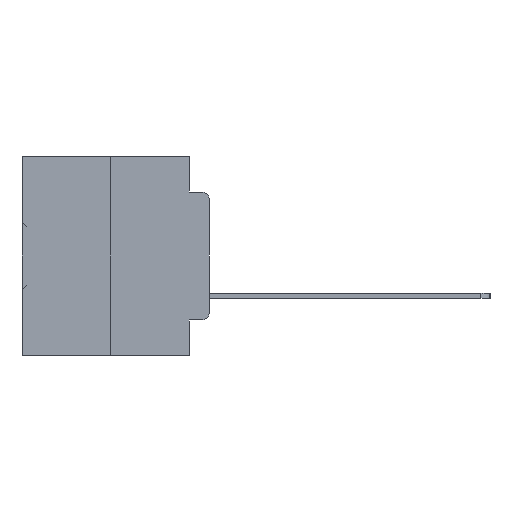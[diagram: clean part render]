
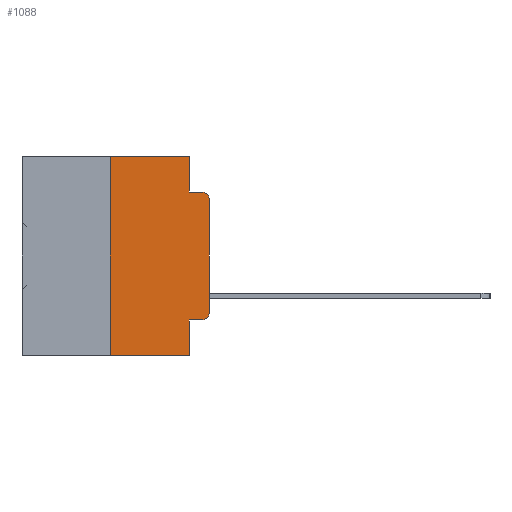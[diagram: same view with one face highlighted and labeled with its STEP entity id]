
A CAD part, left-side view. The second image highlights one B-rep face of the part: STEP entity #1088.
In plain terms, the highlighted planar face has unit normal (-1, 0, 0).
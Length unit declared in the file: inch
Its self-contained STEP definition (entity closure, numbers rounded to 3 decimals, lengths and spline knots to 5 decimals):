
#59 = VECTOR ( 'NONE', #17079, 39.37008 ) ;
#864 = VERTEX_POINT ( 'NONE', #17321 ) ;
#1088 = ADVANCED_FACE ( 'NONE', ( #10720 ), #14314, .F. ) ;
#1730 = EDGE_CURVE ( 'NONE', #35732, #24740, #2333, .T. ) ;
#1788 = VERTEX_POINT ( 'NONE', #37149 ) ;
#1879 = CARTESIAN_POINT ( 'NONE',  ( 0., 0.051, 0. ) ) ;
#2210 = CARTESIAN_POINT ( 'NONE',  ( 0., 0.473, -0.5 ) ) ;
#2333 = CIRCLE ( 'NONE', #30928, 0.02 ) ;
#2561 = CARTESIAN_POINT ( 'NONE',  ( 0., 0.02, -0.4115 ) ) ;
#2634 = CARTESIAN_POINT ( 'NONE',  ( 0., 0.02, -0.1085 ) ) ;
#4165 = CARTESIAN_POINT ( 'NONE',  ( 0., 0.051, -0.4115 ) ) ;
#4414 = ORIENTED_EDGE ( 'NONE', *, *, #24298, .T. ) ;
#4488 = CARTESIAN_POINT ( 'NONE',  ( 0., 0., -0.1085 ) ) ;
#5608 = DIRECTION ( 'NONE',  ( 0., 0., -1. ) ) ;
#6317 = ORIENTED_EDGE ( 'NONE', *, *, #7487, .T. ) ;
#6856 = DIRECTION ( 'NONE',  ( 0., -1., 0. ) ) ;
#7487 = EDGE_CURVE ( 'NONE', #1788, #19315, #37356, .T. ) ;
#7674 = CARTESIAN_POINT ( 'NONE',  ( 0., 0., -0.3915 ) ) ;
#8418 = VECTOR ( 'NONE', #15881, 39.37008 ) ;
#8560 = VERTEX_POINT ( 'NONE', #4488 ) ;
#8838 = CARTESIAN_POINT ( 'NONE',  ( 0., 0., 0. ) ) ;
#9308 = LINE ( 'NONE', #24654, #8418 ) ;
#9413 = VECTOR ( 'NONE', #15816, 39.37008 ) ;
#9637 = ORIENTED_EDGE ( 'NONE', *, *, #1730, .T. ) ;
#10370 = EDGE_CURVE ( 'NONE', #1788, #12035, #9308, .T. ) ;
#10548 = ORIENTED_EDGE ( 'NONE', *, *, #35465, .F. ) ;
#10720 = FACE_OUTER_BOUND ( 'NONE', #19224, .T. ) ;
#12035 = VERTEX_POINT ( 'NONE', #26946 ) ;
#12354 = ORIENTED_EDGE ( 'NONE', *, *, #37311, .T. ) ;
#12417 = LINE ( 'NONE', #8838, #26954 ) ;
#14092 = CARTESIAN_POINT ( 'NONE',  ( 0., 0.051, -0.0885 ) ) ;
#14259 = VERTEX_POINT ( 'NONE', #27947 ) ;
#14281 = AXIS2_PLACEMENT_3D ( 'NONE', #2634, #23186, #5608 ) ;
#14314 = PLANE ( 'NONE',  #16425 ) ;
#14421 = VECTOR ( 'NONE', #6856, 39.37008 ) ;
#14542 = VECTOR ( 'NONE', #18047, 39.37008 ) ;
#15339 = LINE ( 'NONE', #30090, #14421 ) ;
#15689 = LINE ( 'NONE', #14092, #59 ) ;
#15816 = DIRECTION ( 'NONE',  ( 0., -1., 0. ) ) ;
#15881 = DIRECTION ( 'NONE',  ( 0., 0., 1. ) ) ;
#16292 = EDGE_CURVE ( 'NONE', #27355, #19315, #27420, .T. ) ;
#16425 = AXIS2_PLACEMENT_3D ( 'NONE', #20991, #34455, #35782 ) ;
#16522 = EDGE_CURVE ( 'NONE', #24740, #8560, #12417, .T. ) ;
#17079 = DIRECTION ( 'NONE',  ( 0., -1., 0. ) ) ;
#17321 = CARTESIAN_POINT ( 'NONE',  ( 0., 0.02, -0.0885 ) ) ;
#18047 = DIRECTION ( 'NONE',  ( 0., -1., 0. ) ) ;
#18941 = EDGE_CURVE ( 'NONE', #14259, #30558, #26630, .T. ) ;
#19224 = EDGE_LOOP ( 'NONE', ( #26865, #4414, #21924, #26434, #10548, #26854, #6317, #25113, #12354, #9637 ) ) ;
#19315 = VERTEX_POINT ( 'NONE', #29907 ) ;
#19496 = CARTESIAN_POINT ( 'NONE',  ( 0., 0.051, 0. ) ) ;
#19662 = EDGE_CURVE ( 'NONE', #30558, #864, #15689, .T. ) ;
#20991 = CARTESIAN_POINT ( 'NONE',  ( 0., 0.473, 0. ) ) ;
#21924 = ORIENTED_EDGE ( 'NONE', *, *, #19662, .F. ) ;
#22443 = DIRECTION ( 'NONE',  ( 0., 0., -1. ) ) ;
#23186 = DIRECTION ( 'NONE',  ( -1., 0., 0. ) ) ;
#23424 = DIRECTION ( 'NONE',  ( 0., 0., 1. ) ) ;
#24298 = EDGE_CURVE ( 'NONE', #8560, #864, #32648, .T. ) ;
#24654 = CARTESIAN_POINT ( 'NONE',  ( 0., 0.25, 0. ) ) ;
#24740 = VERTEX_POINT ( 'NONE', #7674 ) ;
#24969 = LINE ( 'NONE', #30186, #9413 ) ;
#25113 = ORIENTED_EDGE ( 'NONE', *, *, #16292, .F. ) ;
#25360 = DIRECTION ( 'NONE',  ( -1., 0., 0. ) ) ;
#26434 = ORIENTED_EDGE ( 'NONE', *, *, #18941, .F. ) ;
#26630 = LINE ( 'NONE', #19496, #33259 ) ;
#26854 = ORIENTED_EDGE ( 'NONE', *, *, #10370, .F. ) ;
#26865 = ORIENTED_EDGE ( 'NONE', *, *, #16522, .T. ) ;
#26946 = CARTESIAN_POINT ( 'NONE',  ( 0., 0.25, 0. ) ) ;
#26954 = VECTOR ( 'NONE', #23424, 39.37008 ) ;
#27355 = VERTEX_POINT ( 'NONE', #4165 ) ;
#27420 = LINE ( 'NONE', #1879, #34025 ) ;
#27947 = CARTESIAN_POINT ( 'NONE',  ( 0., 0.051, 0. ) ) ;
#28173 = DIRECTION ( 'NONE',  ( 0., 0., -1. ) ) ;
#28335 = CARTESIAN_POINT ( 'NONE',  ( 0., 0.02, -0.3915 ) ) ;
#29907 = CARTESIAN_POINT ( 'NONE',  ( 0., 0.051, -0.5 ) ) ;
#30090 = CARTESIAN_POINT ( 'NONE',  ( 0., 0.473, 0. ) ) ;
#30186 = CARTESIAN_POINT ( 'NONE',  ( 0., 0.051, -0.4115 ) ) ;
#30558 = VERTEX_POINT ( 'NONE', #31582 ) ;
#30928 = AXIS2_PLACEMENT_3D ( 'NONE', #28335, #25360, #34035 ) ;
#31582 = CARTESIAN_POINT ( 'NONE',  ( 0., 0.051, -0.0885 ) ) ;
#32648 = CIRCLE ( 'NONE', #14281, 0.02 ) ;
#33259 = VECTOR ( 'NONE', #22443, 39.37008 ) ;
#34025 = VECTOR ( 'NONE', #28173, 39.37008 ) ;
#34035 = DIRECTION ( 'NONE',  ( 0., 0., -1. ) ) ;
#34455 = DIRECTION ( 'NONE',  ( 1., 0., 0. ) ) ;
#35465 = EDGE_CURVE ( 'NONE', #12035, #14259, #15339, .T. ) ;
#35732 = VERTEX_POINT ( 'NONE', #2561 ) ;
#35782 = DIRECTION ( 'NONE',  ( 0., 0., -1. ) ) ;
#37149 = CARTESIAN_POINT ( 'NONE',  ( 0., 0.25, -0.5 ) ) ;
#37311 = EDGE_CURVE ( 'NONE', #27355, #35732, #24969, .T. ) ;
#37356 = LINE ( 'NONE', #2210, #14542 ) ;
